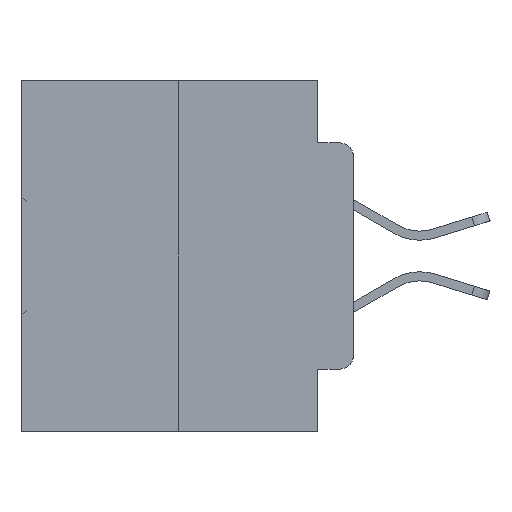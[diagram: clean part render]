
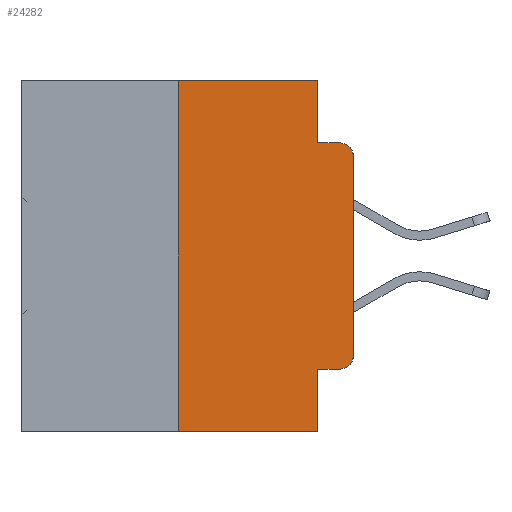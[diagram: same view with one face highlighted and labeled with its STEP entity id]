
A CAD part, left-side view. The second image highlights one B-rep face of the part: STEP entity #24282.
In plain terms, the highlighted planar face has unit normal (-1, 0, 0).
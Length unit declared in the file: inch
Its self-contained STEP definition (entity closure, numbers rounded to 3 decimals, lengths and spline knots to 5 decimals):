
#529 = DIRECTION ( 'NONE',  ( 0., 0., -1. ) ) ;
#686 = VECTOR ( 'NONE', #22700, 39.37008 ) ;
#983 = CIRCLE ( 'NONE', #33035, 0.02 ) ;
#1063 = VECTOR ( 'NONE', #33722, 39.37008 ) ;
#1170 = ORIENTED_EDGE ( 'NONE', *, *, #25855, .T. ) ;
#1551 = LINE ( 'NONE', #20018, #686 ) ;
#2364 = VERTEX_POINT ( 'NONE', #25071 ) ;
#2410 = EDGE_CURVE ( 'NONE', #23388, #31565, #983, .T. ) ;
#2600 = DIRECTION ( 'NONE',  ( 0., 0., -1. ) ) ;
#2771 = LINE ( 'NONE', #3714, #30185 ) ;
#3714 = CARTESIAN_POINT ( 'NONE',  ( 0., 0.051, 0. ) ) ;
#3853 = VERTEX_POINT ( 'NONE', #12934 ) ;
#3952 = LINE ( 'NONE', #21850, #30531 ) ;
#4001 = CARTESIAN_POINT ( 'NONE',  ( 0., 0.051, -0.5 ) ) ;
#4417 = CARTESIAN_POINT ( 'NONE',  ( 0., 0.051, -0.4115 ) ) ;
#4848 = CARTESIAN_POINT ( 'NONE',  ( 0., 0.473, -0.5 ) ) ;
#5394 = LINE ( 'NONE', #10153, #32795 ) ;
#6077 = EDGE_LOOP ( 'NONE', ( #33188, #1170, #7758, #24016, #19551, #25743, #6683, #10065, #15907, #28111 ) ) ;
#6571 = CARTESIAN_POINT ( 'NONE',  ( 0., 0.25, 0. ) ) ;
#6683 = ORIENTED_EDGE ( 'NONE', *, *, #14487, .T. ) ;
#7112 = CARTESIAN_POINT ( 'NONE',  ( 0., 0.051, -0.0885 ) ) ;
#7758 = ORIENTED_EDGE ( 'NONE', *, *, #29805, .F. ) ;
#7791 = VECTOR ( 'NONE', #8435, 39.37008 ) ;
#7930 = VERTEX_POINT ( 'NONE', #30525 ) ;
#8299 = LINE ( 'NONE', #4417, #14587 ) ;
#8435 = DIRECTION ( 'NONE',  ( 0., 0., 1. ) ) ;
#8562 = VERTEX_POINT ( 'NONE', #6571 ) ;
#9017 = LINE ( 'NONE', #33146, #1063 ) ;
#9324 = VERTEX_POINT ( 'NONE', #7112 ) ;
#9700 = DIRECTION ( 'NONE',  ( 0., -1., 0. ) ) ;
#10065 = ORIENTED_EDGE ( 'NONE', *, *, #33248, .F. ) ;
#10153 = CARTESIAN_POINT ( 'NONE',  ( 0., 0.25, 0. ) ) ;
#11994 = VERTEX_POINT ( 'NONE', #12352 ) ;
#12251 = EDGE_CURVE ( 'NONE', #11994, #9324, #3952, .T. ) ;
#12352 = CARTESIAN_POINT ( 'NONE',  ( 0., 0.051, 0. ) ) ;
#12456 = CARTESIAN_POINT ( 'NONE',  ( 0., 0.02, -0.1085 ) ) ;
#12767 = FACE_OUTER_BOUND ( 'NONE', #6077, .T. ) ;
#12934 = CARTESIAN_POINT ( 'NONE',  ( 0., 0.051, -0.4115 ) ) ;
#13226 = PLANE ( 'NONE',  #22750 ) ;
#14486 = DIRECTION ( 'NONE',  ( 0., 0., -1. ) ) ;
#14487 = EDGE_CURVE ( 'NONE', #2364, #27073, #29911, .T. ) ;
#14587 = VECTOR ( 'NONE', #9700, 39.37008 ) ;
#14898 = DIRECTION ( 'NONE',  ( -1., 0., 0. ) ) ;
#15157 = DIRECTION ( 'NONE',  ( 0., 0., -1. ) ) ;
#15231 = CIRCLE ( 'NONE', #15241, 0.02 ) ;
#15241 = AXIS2_PLACEMENT_3D ( 'NONE', #12456, #30994, #15157 ) ;
#15907 = ORIENTED_EDGE ( 'NONE', *, *, #27297, .T. ) ;
#16333 = EDGE_CURVE ( 'NONE', #31565, #7930, #21921, .T. ) ;
#17540 = CARTESIAN_POINT ( 'NONE',  ( 0., 0.02, -0.0885 ) ) ;
#18564 = DIRECTION ( 'NONE',  ( 1., 0., 0. ) ) ;
#19551 = ORIENTED_EDGE ( 'NONE', *, *, #29138, .F. ) ;
#20018 = CARTESIAN_POINT ( 'NONE',  ( 0., 0.473, 0. ) ) ;
#20777 = DIRECTION ( 'NONE',  ( 0., -1., 0. ) ) ;
#21850 = CARTESIAN_POINT ( 'NONE',  ( 0., 0.051, 0. ) ) ;
#21921 = LINE ( 'NONE', #29644, #7791 ) ;
#22700 = DIRECTION ( 'NONE',  ( 0., -1., 0. ) ) ;
#22750 = AXIS2_PLACEMENT_3D ( 'NONE', #34360, #18564, #2600 ) ;
#23388 = VERTEX_POINT ( 'NONE', #25560 ) ;
#23730 = VECTOR ( 'NONE', #20777, 39.37008 ) ;
#24016 = ORIENTED_EDGE ( 'NONE', *, *, #12251, .F. ) ;
#24282 = ADVANCED_FACE ( 'NONE', ( #12767 ), #13226, .F. ) ;
#24337 = CARTESIAN_POINT ( 'NONE',  ( 0., 0., -0.3915 ) ) ;
#25071 = CARTESIAN_POINT ( 'NONE',  ( 0., 0.25, -0.5 ) ) ;
#25560 = CARTESIAN_POINT ( 'NONE',  ( 0., 0.02, -0.4115 ) ) ;
#25743 = ORIENTED_EDGE ( 'NONE', *, *, #27383, .F. ) ;
#25855 = EDGE_CURVE ( 'NONE', #7930, #31832, #15231, .T. ) ;
#27073 = VERTEX_POINT ( 'NONE', #4001 ) ;
#27297 = EDGE_CURVE ( 'NONE', #3853, #23388, #8299, .T. ) ;
#27383 = EDGE_CURVE ( 'NONE', #2364, #8562, #5394, .T. ) ;
#28111 = ORIENTED_EDGE ( 'NONE', *, *, #2410, .T. ) ;
#29138 = EDGE_CURVE ( 'NONE', #8562, #11994, #1551, .T. ) ;
#29644 = CARTESIAN_POINT ( 'NONE',  ( 0., 0., 0. ) ) ;
#29805 = EDGE_CURVE ( 'NONE', #9324, #31832, #9017, .T. ) ;
#29911 = LINE ( 'NONE', #4848, #23730 ) ;
#30185 = VECTOR ( 'NONE', #14486, 39.37008 ) ;
#30525 = CARTESIAN_POINT ( 'NONE',  ( 0., 0., -0.1085 ) ) ;
#30531 = VECTOR ( 'NONE', #529, 39.37008 ) ;
#30726 = CARTESIAN_POINT ( 'NONE',  ( 0., 0.02, -0.3915 ) ) ;
#30994 = DIRECTION ( 'NONE',  ( -1., 0., 0. ) ) ;
#31565 = VERTEX_POINT ( 'NONE', #24337 ) ;
#31832 = VERTEX_POINT ( 'NONE', #17540 ) ;
#32795 = VECTOR ( 'NONE', #33991, 39.37008 ) ;
#33035 = AXIS2_PLACEMENT_3D ( 'NONE', #30726, #14898, #33369 ) ;
#33146 = CARTESIAN_POINT ( 'NONE',  ( 0., 0.051, -0.0885 ) ) ;
#33188 = ORIENTED_EDGE ( 'NONE', *, *, #16333, .T. ) ;
#33248 = EDGE_CURVE ( 'NONE', #3853, #27073, #2771, .T. ) ;
#33369 = DIRECTION ( 'NONE',  ( 0., 0., -1. ) ) ;
#33722 = DIRECTION ( 'NONE',  ( 0., -1., 0. ) ) ;
#33991 = DIRECTION ( 'NONE',  ( 0., 0., 1. ) ) ;
#34360 = CARTESIAN_POINT ( 'NONE',  ( 0., 0.473, 0. ) ) ;
